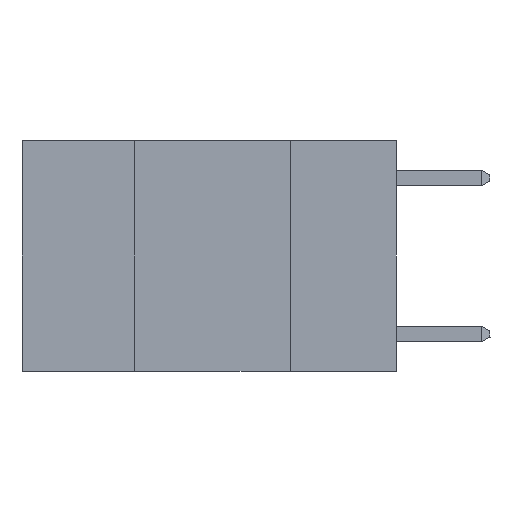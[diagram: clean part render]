
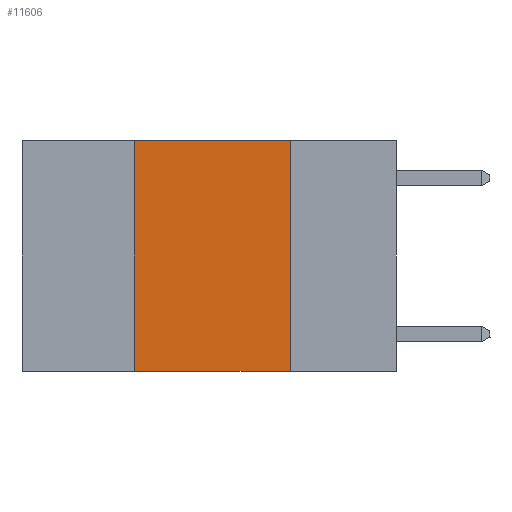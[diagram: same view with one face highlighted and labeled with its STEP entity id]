
A CAD part, left-side view. The second image highlights one B-rep face of the part: STEP entity #11606.
In plain terms, the highlighted planar face has unit normal (-1, 0, 0).
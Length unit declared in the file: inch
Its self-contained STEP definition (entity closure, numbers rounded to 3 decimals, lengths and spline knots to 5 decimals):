
#44 = CARTESIAN_POINT ( 'NONE',  ( 0., 0.17, 0. ) ) ;
#289 = EDGE_CURVE ( 'NONE', #17483, #14474, #343, .T. ) ;
#343 = LINE ( 'NONE', #8789, #11610 ) ;
#2905 = DIRECTION ( 'NONE',  ( 0., 0., -1. ) ) ;
#3873 = CARTESIAN_POINT ( 'NONE',  ( 0., 0.6, 0. ) ) ;
#4285 = VECTOR ( 'NONE', #17159, 39.37008 ) ;
#4962 = CARTESIAN_POINT ( 'NONE',  ( 0., 0.6, 0. ) ) ;
#5008 = VERTEX_POINT ( 'NONE', #7321 ) ;
#6398 = DIRECTION ( 'NONE',  ( 1., 0., 0. ) ) ;
#7128 = ORIENTED_EDGE ( 'NONE', *, *, #13141, .F. ) ;
#7199 = AXIS2_PLACEMENT_3D ( 'NONE', #4962, #6398, #16417 ) ;
#7321 = CARTESIAN_POINT ( 'NONE',  ( 0., 0.42, -0.37 ) ) ;
#7350 = EDGE_CURVE ( 'NONE', #5008, #11644, #16092, .T. ) ;
#8789 = CARTESIAN_POINT ( 'NONE',  ( 0., 0.17, 0. ) ) ;
#10392 = FACE_OUTER_BOUND ( 'NONE', #17516, .T. ) ;
#10628 = CARTESIAN_POINT ( 'NONE',  ( 0., 0.17, -0.37 ) ) ;
#10832 = EDGE_CURVE ( 'NONE', #5008, #14474, #12020, .T. ) ;
#11606 = ADVANCED_FACE ( 'NONE', ( #10392 ), #13607, .F. ) ;
#11610 = VECTOR ( 'NONE', #2905, 39.37008 ) ;
#11644 = VERTEX_POINT ( 'NONE', #15068 ) ;
#11944 = ORIENTED_EDGE ( 'NONE', *, *, #10832, .T. ) ;
#12020 = LINE ( 'NONE', #15731, #4285 ) ;
#12732 = CARTESIAN_POINT ( 'NONE',  ( 0., 0.42, 0. ) ) ;
#13141 = EDGE_CURVE ( 'NONE', #11644, #17483, #18087, .T. ) ;
#13607 = PLANE ( 'NONE',  #7199 ) ;
#13903 = ORIENTED_EDGE ( 'NONE', *, *, #289, .F. ) ;
#14141 = DIRECTION ( 'NONE',  ( 0., 0., 1. ) ) ;
#14340 = VECTOR ( 'NONE', #18242, 39.37008 ) ;
#14474 = VERTEX_POINT ( 'NONE', #10628 ) ;
#14795 = ORIENTED_EDGE ( 'NONE', *, *, #7350, .F. ) ;
#15068 = CARTESIAN_POINT ( 'NONE',  ( 0., 0.42, 0. ) ) ;
#15631 = VECTOR ( 'NONE', #14141, 39.37008 ) ;
#15731 = CARTESIAN_POINT ( 'NONE',  ( 0., 0.6, -0.37 ) ) ;
#16092 = LINE ( 'NONE', #12732, #15631 ) ;
#16417 = DIRECTION ( 'NONE',  ( 0., 0., -1. ) ) ;
#17159 = DIRECTION ( 'NONE',  ( 0., -1., 0. ) ) ;
#17483 = VERTEX_POINT ( 'NONE', #44 ) ;
#17516 = EDGE_LOOP ( 'NONE', ( #13903, #7128, #14795, #11944 ) ) ;
#18087 = LINE ( 'NONE', #3873, #14340 ) ;
#18242 = DIRECTION ( 'NONE',  ( 0., -1., 0. ) ) ;
